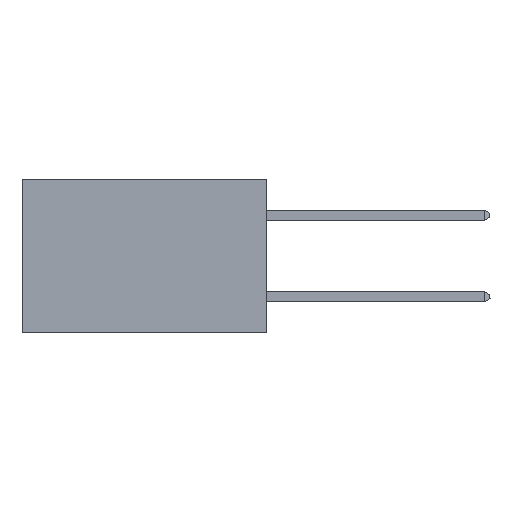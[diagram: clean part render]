
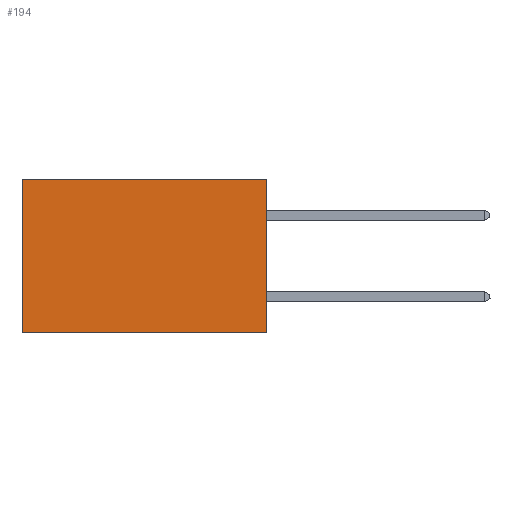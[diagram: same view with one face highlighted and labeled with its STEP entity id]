
A CAD part, left-side view. The second image highlights one B-rep face of the part: STEP entity #194.
In plain terms, the highlighted planar face has unit normal (-1, 0, 0).
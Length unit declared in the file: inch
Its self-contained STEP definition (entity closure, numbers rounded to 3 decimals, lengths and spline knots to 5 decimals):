
#194 = ADVANCED_FACE ( 'NONE', ( #5339 ), #12959, .F. ) ;
#257 = VECTOR ( 'NONE', #18715, 39.37008 ) ;
#839 = VERTEX_POINT ( 'NONE', #9470 ) ;
#1364 = DIRECTION ( 'NONE',  ( 0., 0., -1. ) ) ;
#1892 = DIRECTION ( 'NONE',  ( 0., 1., 0. ) ) ;
#1960 = EDGE_CURVE ( 'NONE', #12340, #7831, #16748, .T. ) ;
#3212 = CARTESIAN_POINT ( 'NONE',  ( 0.2875, 0.6, -0.375 ) ) ;
#4794 = CARTESIAN_POINT ( 'NONE',  ( 0.2875, 0., -0.375 ) ) ;
#5339 = FACE_OUTER_BOUND ( 'NONE', #21104, .T. ) ;
#5842 = EDGE_CURVE ( 'NONE', #11180, #839, #16075, .T. ) ;
#5940 = LINE ( 'NONE', #19808, #20853 ) ;
#6082 = CARTESIAN_POINT ( 'NONE',  ( 0.2875, 0., -0.375 ) ) ;
#6146 = DIRECTION ( 'NONE',  ( 1., 0., 0. ) ) ;
#6533 = EDGE_CURVE ( 'NONE', #12340, #11180, #5940, .T. ) ;
#7297 = ORIENTED_EDGE ( 'NONE', *, *, #5842, .F. ) ;
#7634 = ORIENTED_EDGE ( 'NONE', *, *, #14829, .T. ) ;
#7654 = CARTESIAN_POINT ( 'NONE',  ( 0.2875, 0.6, 0. ) ) ;
#7745 = LINE ( 'NONE', #3212, #16584 ) ;
#7831 = VERTEX_POINT ( 'NONE', #7654 ) ;
#7943 = CARTESIAN_POINT ( 'NONE',  ( 0.2875, 0., 0. ) ) ;
#9244 = ORIENTED_EDGE ( 'NONE', *, *, #6533, .F. ) ;
#9337 = AXIS2_PLACEMENT_3D ( 'NONE', #6082, #6146, #19580 ) ;
#9470 = CARTESIAN_POINT ( 'NONE',  ( 0.2875, 0.6, -0.375 ) ) ;
#11180 = VERTEX_POINT ( 'NONE', #4794 ) ;
#12340 = VERTEX_POINT ( 'NONE', #7943 ) ;
#12959 = PLANE ( 'NONE',  #9337 ) ;
#14621 = ORIENTED_EDGE ( 'NONE', *, *, #1960, .T. ) ;
#14829 = EDGE_CURVE ( 'NONE', #7831, #839, #7745, .T. ) ;
#14934 = DIRECTION ( 'NONE',  ( 0., 0., -1. ) ) ;
#15018 = VECTOR ( 'NONE', #1892, 39.37008 ) ;
#16075 = LINE ( 'NONE', #20128, #15018 ) ;
#16584 = VECTOR ( 'NONE', #14934, 39.37008 ) ;
#16748 = LINE ( 'NONE', #17033, #257 ) ;
#17033 = CARTESIAN_POINT ( 'NONE',  ( 0.2875, 0., 0. ) ) ;
#18715 = DIRECTION ( 'NONE',  ( 0., 1., 0. ) ) ;
#19580 = DIRECTION ( 'NONE',  ( 0., 0., -1. ) ) ;
#19808 = CARTESIAN_POINT ( 'NONE',  ( 0.2875, 0., -0.375 ) ) ;
#20128 = CARTESIAN_POINT ( 'NONE',  ( 0.2875, 0., -0.375 ) ) ;
#20853 = VECTOR ( 'NONE', #1364, 39.37008 ) ;
#21104 = EDGE_LOOP ( 'NONE', ( #7634, #7297, #9244, #14621 ) ) ;
